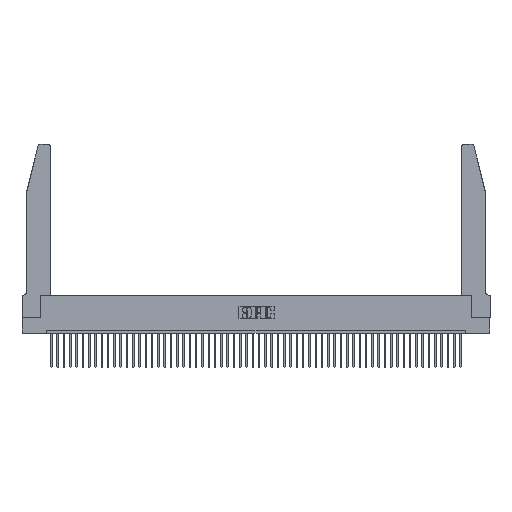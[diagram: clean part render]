
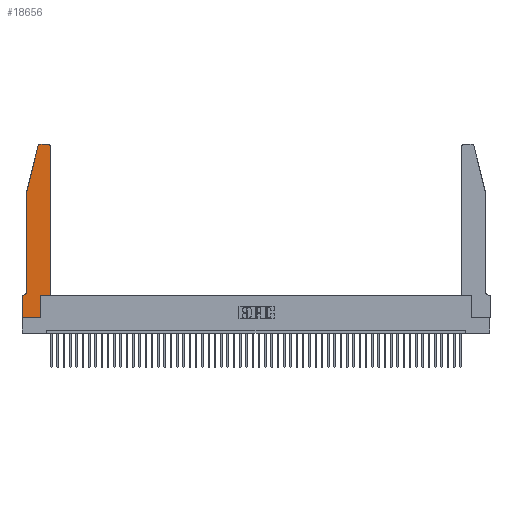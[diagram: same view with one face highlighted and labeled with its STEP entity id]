
A CAD part, top view. The second image highlights one B-rep face of the part: STEP entity #18656.
In plain terms, the highlighted planar face has unit normal (0, 0, 1).
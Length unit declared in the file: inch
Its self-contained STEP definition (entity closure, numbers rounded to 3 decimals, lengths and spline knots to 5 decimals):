
#535 = VECTOR ( 'NONE', #21957, 39.37008 ) ;
#1089 = CARTESIAN_POINT ( 'NONE',  ( 0.2605, 2.75, 0.37 ) ) ;
#1590 = ORIENTED_EDGE ( 'NONE', *, *, #40266, .T. ) ;
#2395 = DIRECTION ( 'NONE',  ( 0., 0., -1. ) ) ;
#2753 = VECTOR ( 'NONE', #29144, 39.37008 ) ;
#3239 = DIRECTION ( 'NONE',  ( 0., 0., 1. ) ) ;
#3383 = ORIENTED_EDGE ( 'NONE', *, *, #42591, .T. ) ;
#3804 = CARTESIAN_POINT ( 'NONE',  ( 0.0755, 2., 0.37 ) ) ;
#3968 = LINE ( 'NONE', #35973, #42298 ) ;
#4667 = CARTESIAN_POINT ( 'NONE',  ( 0.4205, 2.75, 0.37 ) ) ;
#5518 = LINE ( 'NONE', #45770, #535 ) ;
#5549 = LINE ( 'NONE', #3804, #38967 ) ;
#6120 = EDGE_CURVE ( 'NONE', #8825, #30728, #23201, .T. ) ;
#6356 = DIRECTION ( 'NONE',  ( -1., 0., 0. ) ) ;
#6486 = CIRCLE ( 'NONE', #32284, 0.03 ) ;
#6645 = EDGE_CURVE ( 'NONE', #50118, #12574, #3968, .T. ) ;
#6778 = DIRECTION ( 'NONE',  ( 1., 0., 0. ) ) ;
#7069 = LINE ( 'NONE', #33435, #2753 ) ;
#7600 = LINE ( 'NONE', #37525, #25417 ) ;
#8696 = DIRECTION ( 'NONE',  ( 0., -1., 0. ) ) ;
#8709 = DIRECTION ( 'NONE',  ( -1., 0., 0. ) ) ;
#8825 = VERTEX_POINT ( 'NONE', #49502 ) ;
#8887 = VECTOR ( 'NONE', #43394, 39.37008 ) ;
#8936 = VERTEX_POINT ( 'NONE', #13654 ) ;
#8974 = ORIENTED_EDGE ( 'NONE', *, *, #40145, .T. ) ;
#9014 = VECTOR ( 'NONE', #8696, 39.37008 ) ;
#9810 = AXIS2_PLACEMENT_3D ( 'NONE', #26245, #35052, #46626 ) ;
#10254 = ORIENTED_EDGE ( 'NONE', *, *, #17724, .T. ) ;
#11524 = LINE ( 'NONE', #25670, #9014 ) ;
#11675 = DIRECTION ( 'NONE',  ( 0., -1., 0. ) ) ;
#11750 = EDGE_CURVE ( 'NONE', #8936, #38489, #48715, .T. ) ;
#12574 = VERTEX_POINT ( 'NONE', #50200 ) ;
#13096 = VERTEX_POINT ( 'NONE', #15031 ) ;
#13373 = VECTOR ( 'NONE', #8709, 39.37008 ) ;
#13654 = CARTESIAN_POINT ( 'NONE',  ( 0., 0., 0.37 ) ) ;
#15031 = CARTESIAN_POINT ( 'NONE',  ( 0.25487, 2.72718, 0.37 ) ) ;
#15575 = DIRECTION ( 'NONE',  ( -0.239, -0.971, 0. ) ) ;
#17724 = EDGE_CURVE ( 'NONE', #37174, #18809, #6486, .T. ) ;
#17735 = DIRECTION ( 'NONE',  ( 1., 0., 0. ) ) ;
#18263 = ORIENTED_EDGE ( 'NONE', *, *, #6645, .T. ) ;
#18656 = ADVANCED_FACE ( 'NONE', ( #50855 ), #45742, .T. ) ;
#18809 = VERTEX_POINT ( 'NONE', #4667 ) ;
#19770 = ORIENTED_EDGE ( 'NONE', *, *, #33294, .T. ) ;
#19984 = CARTESIAN_POINT ( 'NONE',  ( 0.4505, 2.72, 0.37 ) ) ;
#20742 = VERTEX_POINT ( 'NONE', #21209 ) ;
#21146 = CARTESIAN_POINT ( 'NONE',  ( 0.284, 2.72, 0.37 ) ) ;
#21209 = CARTESIAN_POINT ( 'NONE',  ( 0.284, 2.75, 0.37 ) ) ;
#21402 = EDGE_CURVE ( 'NONE', #18809, #20742, #49909, .T. ) ;
#21957 = DIRECTION ( 'NONE',  ( 0., 1., 0. ) ) ;
#22358 = CARTESIAN_POINT ( 'NONE',  ( 0.2865, 0.35, 0.37 ) ) ;
#23201 = LINE ( 'NONE', #39443, #8887 ) ;
#24648 = VECTOR ( 'NONE', #6778, 39.37008 ) ;
#25298 = CARTESIAN_POINT ( 'NONE',  ( 0., 0., 0.37 ) ) ;
#25417 = VECTOR ( 'NONE', #49604, 39.37008 ) ;
#25440 = EDGE_CURVE ( 'NONE', #13096, #50118, #5549, .T. ) ;
#25670 = CARTESIAN_POINT ( 'NONE',  ( 0., 0., 0.37 ) ) ;
#26245 = CARTESIAN_POINT ( 'NONE',  ( 0., 0.35, 0.37 ) ) ;
#27140 = VERTEX_POINT ( 'NONE', #22358 ) ;
#29144 = DIRECTION ( 'NONE',  ( 1., 0., 0. ) ) ;
#30023 = CARTESIAN_POINT ( 'NONE',  ( 0.0055, 0.42, 0.37 ) ) ;
#30068 = VERTEX_POINT ( 'NONE', #31514 ) ;
#30558 = CARTESIAN_POINT ( 'NONE',  ( 0.2865, 0., 0.37 ) ) ;
#30728 = VERTEX_POINT ( 'NONE', #47460 ) ;
#30761 = EDGE_CURVE ( 'NONE', #30728, #8936, #11524, .T. ) ;
#30921 = DIRECTION ( 'NONE',  ( 1., 0., 0. ) ) ;
#31514 = CARTESIAN_POINT ( 'NONE',  ( 0.4505, 0.35, 0.37 ) ) ;
#31632 = ORIENTED_EDGE ( 'NONE', *, *, #21402, .T. ) ;
#32284 = AXIS2_PLACEMENT_3D ( 'NONE', #49912, #3239, #30921 ) ;
#33159 = ORIENTED_EDGE ( 'NONE', *, *, #6120, .T. ) ;
#33294 = EDGE_CURVE ( 'NONE', #30068, #37174, #7600, .T. ) ;
#33435 = CARTESIAN_POINT ( 'NONE',  ( 0.4505, 0.35, 0.37 ) ) ;
#34197 = AXIS2_PLACEMENT_3D ( 'NONE', #21146, #44961, #17735 ) ;
#34243 = CIRCLE ( 'NONE', #39216, 0.07 ) ;
#34641 = ORIENTED_EDGE ( 'NONE', *, *, #30761, .T. ) ;
#34772 = ORIENTED_EDGE ( 'NONE', *, *, #25440, .T. ) ;
#35052 = DIRECTION ( 'NONE',  ( 0., 0., 1. ) ) ;
#35513 = CARTESIAN_POINT ( 'NONE',  ( 0.0755, 2., 0.37 ) ) ;
#35973 = CARTESIAN_POINT ( 'NONE',  ( 0.0755, 2., 0.37 ) ) ;
#37174 = VERTEX_POINT ( 'NONE', #19984 ) ;
#37525 = CARTESIAN_POINT ( 'NONE',  ( 0.4505, 0.35, 0.37 ) ) ;
#38489 = VERTEX_POINT ( 'NONE', #30558 ) ;
#38917 = CIRCLE ( 'NONE', #34197, 0.03 ) ;
#38967 = VECTOR ( 'NONE', #15575, 39.37008 ) ;
#39141 = EDGE_CURVE ( 'NONE', #20742, #13096, #38917, .T. ) ;
#39216 = AXIS2_PLACEMENT_3D ( 'NONE', #30023, #2395, #6356 ) ;
#39443 = CARTESIAN_POINT ( 'NONE',  ( 0.0755, 0.35, 0.37 ) ) ;
#40145 = EDGE_CURVE ( 'NONE', #27140, #30068, #7069, .T. ) ;
#40266 = EDGE_CURVE ( 'NONE', #12574, #8825, #34243, .T. ) ;
#42184 = EDGE_LOOP ( 'NONE', ( #31632, #46950, #34772, #18263, #1590, #33159, #34641, #42420, #3383, #8974, #19770, #10254 ) ) ;
#42298 = VECTOR ( 'NONE', #11675, 39.37008 ) ;
#42420 = ORIENTED_EDGE ( 'NONE', *, *, #11750, .T. ) ;
#42591 = EDGE_CURVE ( 'NONE', #38489, #27140, #5518, .T. ) ;
#43394 = DIRECTION ( 'NONE',  ( -1., 0., 0. ) ) ;
#44961 = DIRECTION ( 'NONE',  ( 0., 0., 1. ) ) ;
#45742 = PLANE ( 'NONE',  #9810 ) ;
#45770 = CARTESIAN_POINT ( 'NONE',  ( 0.2865, 0.35, 0.37 ) ) ;
#46626 = DIRECTION ( 'NONE',  ( 1., 0., 0. ) ) ;
#46950 = ORIENTED_EDGE ( 'NONE', *, *, #39141, .T. ) ;
#47460 = CARTESIAN_POINT ( 'NONE',  ( 0., 0.35, 0.37 ) ) ;
#48715 = LINE ( 'NONE', #25298, #24648 ) ;
#49502 = CARTESIAN_POINT ( 'NONE',  ( 0.0055, 0.35, 0.37 ) ) ;
#49604 = DIRECTION ( 'NONE',  ( 0., 1., 0. ) ) ;
#49909 = LINE ( 'NONE', #1089, #13373 ) ;
#49912 = CARTESIAN_POINT ( 'NONE',  ( 0.4205, 2.72, 0.37 ) ) ;
#50118 = VERTEX_POINT ( 'NONE', #35513 ) ;
#50200 = CARTESIAN_POINT ( 'NONE',  ( 0.0755, 0.42, 0.37 ) ) ;
#50855 = FACE_OUTER_BOUND ( 'NONE', #42184, .T. ) ;
